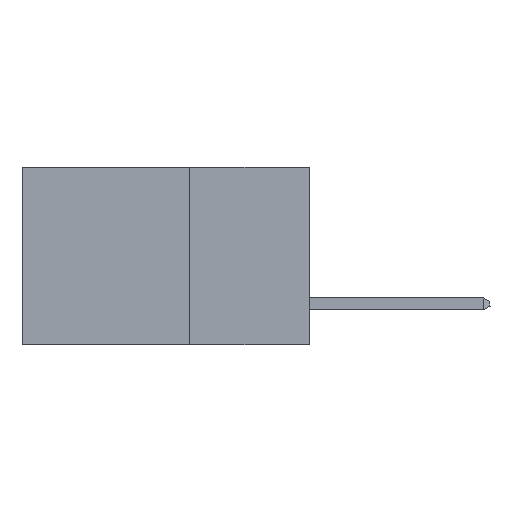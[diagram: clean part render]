
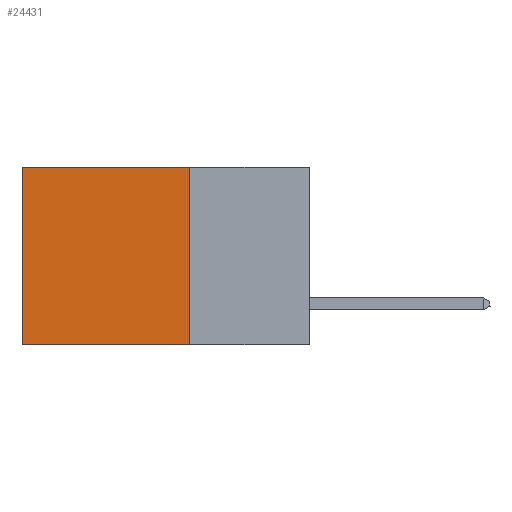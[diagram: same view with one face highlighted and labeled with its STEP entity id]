
A CAD part, left-side view. The second image highlights one B-rep face of the part: STEP entity #24431.
In plain terms, the highlighted planar face has unit normal (-1, 0, 0).
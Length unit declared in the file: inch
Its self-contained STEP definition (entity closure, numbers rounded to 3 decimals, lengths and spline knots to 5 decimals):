
#889 = ORIENTED_EDGE ( 'NONE', *, *, #13242, .F. ) ;
#1411 = CARTESIAN_POINT ( 'NONE',  ( 0.2875, 0.25, 0. ) ) ;
#1532 = PLANE ( 'NONE',  #30026 ) ;
#1984 = FACE_OUTER_BOUND ( 'NONE', #11509, .T. ) ;
#6717 = ORIENTED_EDGE ( 'NONE', *, *, #9846, .T. ) ;
#6718 = VERTEX_POINT ( 'NONE', #17209 ) ;
#7199 = LINE ( 'NONE', #20237, #27597 ) ;
#8197 = VECTOR ( 'NONE', #32485, 39.37008 ) ;
#8654 = VECTOR ( 'NONE', #11856, 39.37008 ) ;
#9846 = EDGE_CURVE ( 'NONE', #10478, #21207, #39376, .T. ) ;
#10478 = VERTEX_POINT ( 'NONE', #32399 ) ;
#11509 = EDGE_LOOP ( 'NONE', ( #6717, #12093, #889, #28648 ) ) ;
#11592 = LINE ( 'NONE', #20954, #8654 ) ;
#11856 = DIRECTION ( 'NONE',  ( 0., 0., -1. ) ) ;
#12093 = ORIENTED_EDGE ( 'NONE', *, *, #18153, .F. ) ;
#13242 = EDGE_CURVE ( 'NONE', #6718, #22167, #11592, .T. ) ;
#17209 = CARTESIAN_POINT ( 'NONE',  ( 0.2875, 0.25, 0. ) ) ;
#17530 = DIRECTION ( 'NONE',  ( 0., 1., 0. ) ) ;
#17754 = CARTESIAN_POINT ( 'NONE',  ( 0.2875, 0.25, -0.37 ) ) ;
#18153 = EDGE_CURVE ( 'NONE', #22167, #21207, #7199, .T. ) ;
#18902 = DIRECTION ( 'NONE',  ( 0., 0., -1. ) ) ;
#20237 = CARTESIAN_POINT ( 'NONE',  ( 0.2875, 0.25, -0.37 ) ) ;
#20954 = CARTESIAN_POINT ( 'NONE',  ( 0.2875, 0.25, 0. ) ) ;
#21207 = VERTEX_POINT ( 'NONE', #37124 ) ;
#22167 = VERTEX_POINT ( 'NONE', #17754 ) ;
#24431 = ADVANCED_FACE ( 'NONE', ( #1984 ), #1532, .F. ) ;
#24710 = CARTESIAN_POINT ( 'NONE',  ( 0.2875, 0.6, 0. ) ) ;
#26204 = CARTESIAN_POINT ( 'NONE',  ( 0.2875, 0.25, 0. ) ) ;
#26696 = DIRECTION ( 'NONE',  ( 0., 0., -1. ) ) ;
#27597 = VECTOR ( 'NONE', #17530, 39.37008 ) ;
#28648 = ORIENTED_EDGE ( 'NONE', *, *, #35846, .T. ) ;
#30026 = AXIS2_PLACEMENT_3D ( 'NONE', #1411, #35843, #26696 ) ;
#31121 = VECTOR ( 'NONE', #18902, 39.37008 ) ;
#32399 = CARTESIAN_POINT ( 'NONE',  ( 0.2875, 0.6, 0. ) ) ;
#32485 = DIRECTION ( 'NONE',  ( 0., 1., 0. ) ) ;
#33956 = LINE ( 'NONE', #26204, #8197 ) ;
#35843 = DIRECTION ( 'NONE',  ( 1., 0., 0. ) ) ;
#35846 = EDGE_CURVE ( 'NONE', #6718, #10478, #33956, .T. ) ;
#37124 = CARTESIAN_POINT ( 'NONE',  ( 0.2875, 0.6, -0.37 ) ) ;
#39376 = LINE ( 'NONE', #24710, #31121 ) ;
